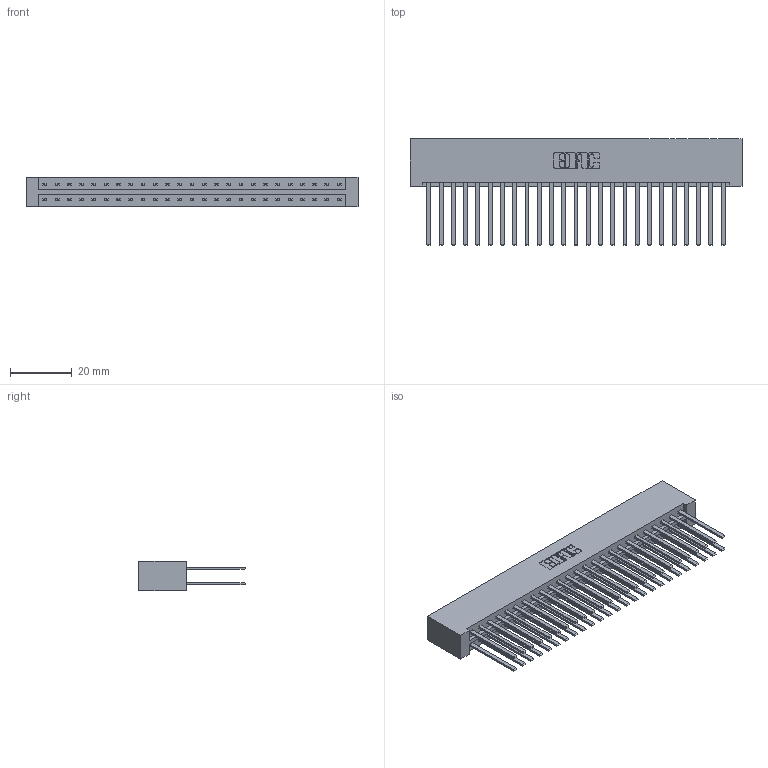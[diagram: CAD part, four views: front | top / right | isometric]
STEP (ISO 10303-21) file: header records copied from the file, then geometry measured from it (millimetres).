
FILE_DESCRIPTION (( 'STEP AP203' ), '1' );
FILE_NAME ('833-050-544-201.STEP', '2020-06-04T17:49:09', ( '' ), ( '' ), 'SwSTEP 2.0', 'SolidWorks 2020', '' );
FILE_SCHEMA (( 'CONFIG_CONTROL_DESIGN' ));
Length unit declared in the file: inch
Products named in the file (3): 833 Part_Lugless; 345-292-001_345-293-144; 833-050-544-201
Assembly tree (51 placements, depth 2):
  833-050-544-201
    833 Part_Lugless
    345-292-001_345-293-144  x50
Bounding box: 107.31 x 34.3 x 9.4 mm (x, y, z)
Volume: 12130.4 mm3; surface area: 16439.6 mm2
Topology: 51 solids, 51 shells, 2406 faces, 7137 edges, 4690 vertices
Faces by surface type: plane 1666, cylinder 740
Entity records: 17821 total; most frequent: CARTESIAN_POINT 2970, ORIENTED_EDGE 2906, DIRECTION 2557, EDGE_CURVE 1453, VECTOR 1337, LINE 1337, VERTEX_POINT 966, AXIS2_PLACEMENT_3D 610
